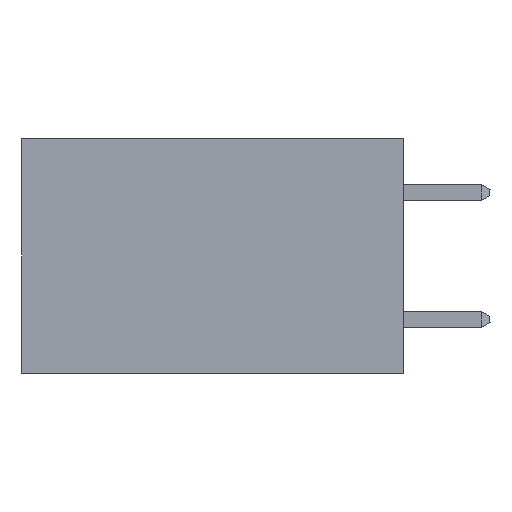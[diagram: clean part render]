
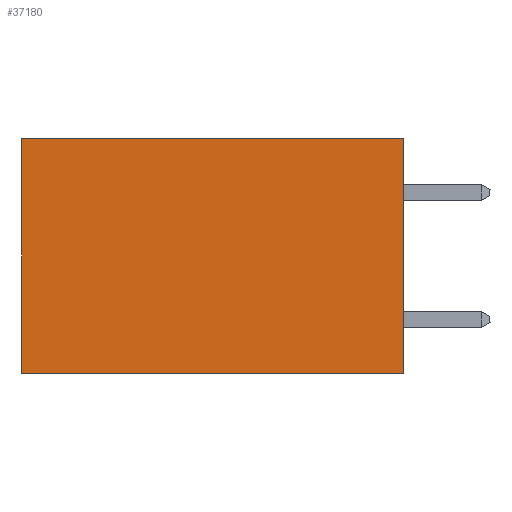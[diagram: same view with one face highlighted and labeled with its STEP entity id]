
A CAD part, left-side view. The second image highlights one B-rep face of the part: STEP entity #37180.
In plain terms, the highlighted planar face has unit normal (-1, 0, 0).
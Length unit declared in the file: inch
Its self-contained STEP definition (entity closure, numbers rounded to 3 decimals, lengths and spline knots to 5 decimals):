
#912 = CARTESIAN_POINT ( 'NONE',  ( 0.2875, 0.6, -0.37 ) ) ;
#1344 = ORIENTED_EDGE ( 'NONE', *, *, #45689, .T. ) ;
#2780 = VERTEX_POINT ( 'NONE', #8990 ) ;
#8990 = CARTESIAN_POINT ( 'NONE',  ( 0.2875, 0., 0. ) ) ;
#9531 = EDGE_CURVE ( 'NONE', #26810, #13846, #34930, .T. ) ;
#10313 = CARTESIAN_POINT ( 'NONE',  ( 0.2875, 0., -0.37 ) ) ;
#10925 = VECTOR ( 'NONE', #24229, 39.37008 ) ;
#13846 = VERTEX_POINT ( 'NONE', #912 ) ;
#15260 = DIRECTION ( 'NONE',  ( 1., 0., 0. ) ) ;
#17499 = DIRECTION ( 'NONE',  ( 0., 1., 0. ) ) ;
#18174 = VERTEX_POINT ( 'NONE', #39540 ) ;
#18364 = EDGE_LOOP ( 'NONE', ( #1344, #36084, #41236, #25299 ) ) ;
#20457 = LINE ( 'NONE', #27550, #10925 ) ;
#22409 = CARTESIAN_POINT ( 'NONE',  ( 0.2875, 0., 0. ) ) ;
#22742 = DIRECTION ( 'NONE',  ( 0., 0., -1. ) ) ;
#22845 = FACE_OUTER_BOUND ( 'NONE', #18364, .T. ) ;
#24229 = DIRECTION ( 'NONE',  ( 0., 0., -1. ) ) ;
#25299 = ORIENTED_EDGE ( 'NONE', *, *, #27927, .T. ) ;
#26073 = CARTESIAN_POINT ( 'NONE',  ( 0.2875, 0., 0. ) ) ;
#26810 = VERTEX_POINT ( 'NONE', #26933 ) ;
#26933 = CARTESIAN_POINT ( 'NONE',  ( 0.2875, 0., -0.37 ) ) ;
#26987 = EDGE_CURVE ( 'NONE', #2780, #26810, #20457, .T. ) ;
#27069 = LINE ( 'NONE', #22409, #39950 ) ;
#27550 = CARTESIAN_POINT ( 'NONE',  ( 0.2875, 0., 0. ) ) ;
#27927 = EDGE_CURVE ( 'NONE', #2780, #18174, #27069, .T. ) ;
#29981 = LINE ( 'NONE', #35019, #38386 ) ;
#30021 = PLANE ( 'NONE',  #41472 ) ;
#33812 = VECTOR ( 'NONE', #17499, 39.37008 ) ;
#34930 = LINE ( 'NONE', #10313, #33812 ) ;
#35019 = CARTESIAN_POINT ( 'NONE',  ( 0.2875, 0.6, 0. ) ) ;
#36084 = ORIENTED_EDGE ( 'NONE', *, *, #9531, .F. ) ;
#37180 = ADVANCED_FACE ( 'NONE', ( #22845 ), #30021, .F. ) ;
#38386 = VECTOR ( 'NONE', #38612, 39.37008 ) ;
#38612 = DIRECTION ( 'NONE',  ( 0., 0., -1. ) ) ;
#39540 = CARTESIAN_POINT ( 'NONE',  ( 0.2875, 0.6, 0. ) ) ;
#39950 = VECTOR ( 'NONE', #43430, 39.37008 ) ;
#41236 = ORIENTED_EDGE ( 'NONE', *, *, #26987, .F. ) ;
#41472 = AXIS2_PLACEMENT_3D ( 'NONE', #26073, #15260, #22742 ) ;
#43430 = DIRECTION ( 'NONE',  ( 0., 1., 0. ) ) ;
#45689 = EDGE_CURVE ( 'NONE', #18174, #13846, #29981, .T. ) ;
